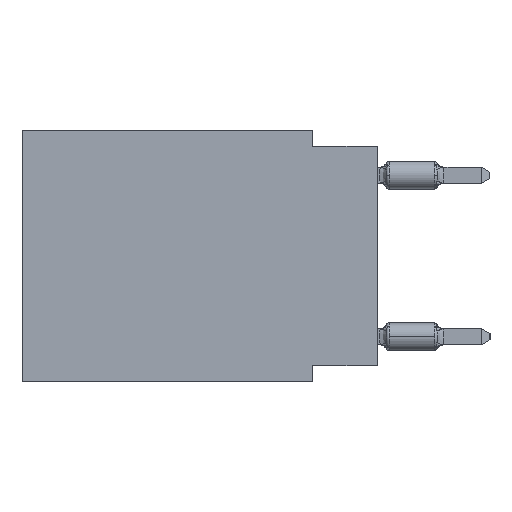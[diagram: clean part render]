
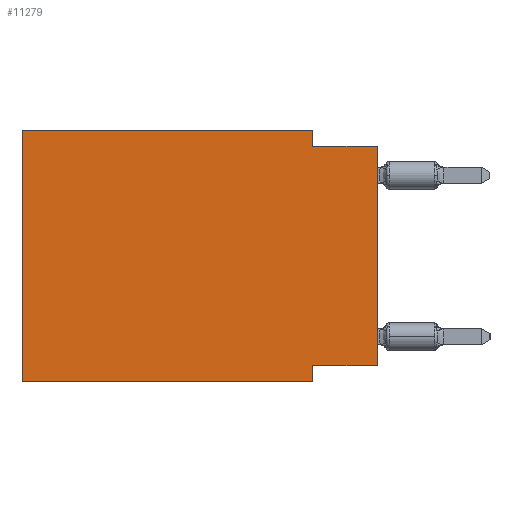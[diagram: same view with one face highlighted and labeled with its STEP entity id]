
A CAD part, left-side view. The second image highlights one B-rep face of the part: STEP entity #11279.
In plain terms, the highlighted planar face has unit normal (-1, 0, 0).
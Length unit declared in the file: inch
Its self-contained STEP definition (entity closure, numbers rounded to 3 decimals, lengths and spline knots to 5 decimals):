
#607 = CARTESIAN_POINT ( 'NONE',  ( 0., 0., -0.025 ) ) ;
#743 = LINE ( 'NONE', #3243, #31086 ) ;
#1059 = LINE ( 'NONE', #21178, #29471 ) ;
#1908 = ORIENTED_EDGE ( 'NONE', *, *, #32560, .F. ) ;
#2328 = CARTESIAN_POINT ( 'NONE',  ( 0., 0.1, -0.025 ) ) ;
#2475 = VECTOR ( 'NONE', #32107, 39.37008 ) ;
#3068 = DIRECTION ( 'NONE',  ( 0., 0., -1. ) ) ;
#3243 = CARTESIAN_POINT ( 'NONE',  ( 0., 0.55, 0. ) ) ;
#4189 = CARTESIAN_POINT ( 'NONE',  ( 0., 0.1, -0.39 ) ) ;
#4243 = ORIENTED_EDGE ( 'NONE', *, *, #20837, .F. ) ;
#5596 = DIRECTION ( 'NONE',  ( 0., 0., -1. ) ) ;
#5980 = CARTESIAN_POINT ( 'NONE',  ( 0., 0., -0.365 ) ) ;
#6203 = EDGE_CURVE ( 'NONE', #25397, #25950, #11549, .T. ) ;
#6693 = ORIENTED_EDGE ( 'NONE', *, *, #29338, .F. ) ;
#6876 = VECTOR ( 'NONE', #17039, 39.37008 ) ;
#7225 = DIRECTION ( 'NONE',  ( 0., -1., 0. ) ) ;
#7669 = ORIENTED_EDGE ( 'NONE', *, *, #14544, .F. ) ;
#8166 = ORIENTED_EDGE ( 'NONE', *, *, #6203, .T. ) ;
#8985 = CARTESIAN_POINT ( 'NONE',  ( 0., 0.55, 0. ) ) ;
#10189 = EDGE_CURVE ( 'NONE', #10452, #11853, #20168, .T. ) ;
#10452 = VERTEX_POINT ( 'NONE', #5980 ) ;
#10866 = DIRECTION ( 'NONE',  ( 0., 1., 0. ) ) ;
#11279 = ADVANCED_FACE ( 'NONE', ( #13949 ), #21668, .F. ) ;
#11549 = LINE ( 'NONE', #22059, #2475 ) ;
#11749 = VECTOR ( 'NONE', #7225, 39.37008 ) ;
#11853 = VERTEX_POINT ( 'NONE', #607 ) ;
#13268 = EDGE_CURVE ( 'NONE', #21883, #25950, #1059, .T. ) ;
#13283 = EDGE_LOOP ( 'NONE', ( #16252, #1908, #22820, #4243, #7669, #8166, #21783, #6693 ) ) ;
#13949 = FACE_OUTER_BOUND ( 'NONE', #13283, .T. ) ;
#14544 = EDGE_CURVE ( 'NONE', #25397, #31404, #743, .T. ) ;
#14718 = LINE ( 'NONE', #17176, #31010 ) ;
#15803 = CARTESIAN_POINT ( 'NONE',  ( 0., 0.1, 0. ) ) ;
#16252 = ORIENTED_EDGE ( 'NONE', *, *, #10189, .T. ) ;
#16569 = DIRECTION ( 'NONE',  ( 1., 0., 0. ) ) ;
#17039 = DIRECTION ( 'NONE',  ( 0., 0., 1. ) ) ;
#17176 = CARTESIAN_POINT ( 'NONE',  ( 0., 0., -0.025 ) ) ;
#17745 = VECTOR ( 'NONE', #10866, 39.37008 ) ;
#18587 = CARTESIAN_POINT ( 'NONE',  ( 0., 0.55, 0. ) ) ;
#19464 = VERTEX_POINT ( 'NONE', #2328 ) ;
#20143 = DIRECTION ( 'NONE',  ( 0., -1., 0. ) ) ;
#20168 = LINE ( 'NONE', #32020, #6876 ) ;
#20837 = EDGE_CURVE ( 'NONE', #31404, #24060, #29466, .T. ) ;
#21178 = CARTESIAN_POINT ( 'NONE',  ( 0., 0.1, -0.39 ) ) ;
#21668 = PLANE ( 'NONE',  #31029 ) ;
#21783 = ORIENTED_EDGE ( 'NONE', *, *, #13268, .F. ) ;
#21883 = VERTEX_POINT ( 'NONE', #23559 ) ;
#22059 = CARTESIAN_POINT ( 'NONE',  ( 0., 0.55, -0.39 ) ) ;
#22820 = ORIENTED_EDGE ( 'NONE', *, *, #29331, .F. ) ;
#23211 = CARTESIAN_POINT ( 'NONE',  ( 0., 0., -0.365 ) ) ;
#23490 = DIRECTION ( 'NONE',  ( 0., 0., 1. ) ) ;
#23559 = CARTESIAN_POINT ( 'NONE',  ( 0., 0.1, -0.365 ) ) ;
#24060 = VERTEX_POINT ( 'NONE', #25627 ) ;
#25397 = VERTEX_POINT ( 'NONE', #30935 ) ;
#25627 = CARTESIAN_POINT ( 'NONE',  ( 0., 0.1, 0. ) ) ;
#25950 = VERTEX_POINT ( 'NONE', #4189 ) ;
#26760 = DIRECTION ( 'NONE',  ( 0., 0., -1. ) ) ;
#26830 = CARTESIAN_POINT ( 'NONE',  ( 0., 0.55, 0. ) ) ;
#28789 = VECTOR ( 'NONE', #5596, 39.37008 ) ;
#29331 = EDGE_CURVE ( 'NONE', #24060, #19464, #31099, .T. ) ;
#29338 = EDGE_CURVE ( 'NONE', #10452, #21883, #30938, .T. ) ;
#29466 = LINE ( 'NONE', #26830, #11749 ) ;
#29471 = VECTOR ( 'NONE', #3068, 39.37008 ) ;
#30935 = CARTESIAN_POINT ( 'NONE',  ( 0., 0.55, -0.39 ) ) ;
#30938 = LINE ( 'NONE', #23211, #17745 ) ;
#31010 = VECTOR ( 'NONE', #20143, 39.37008 ) ;
#31029 = AXIS2_PLACEMENT_3D ( 'NONE', #8985, #16569, #26760 ) ;
#31086 = VECTOR ( 'NONE', #23490, 39.37008 ) ;
#31099 = LINE ( 'NONE', #15803, #28789 ) ;
#31404 = VERTEX_POINT ( 'NONE', #18587 ) ;
#32020 = CARTESIAN_POINT ( 'NONE',  ( 0., 0., 0. ) ) ;
#32107 = DIRECTION ( 'NONE',  ( 0., -1., 0. ) ) ;
#32560 = EDGE_CURVE ( 'NONE', #19464, #11853, #14718, .T. ) ;
